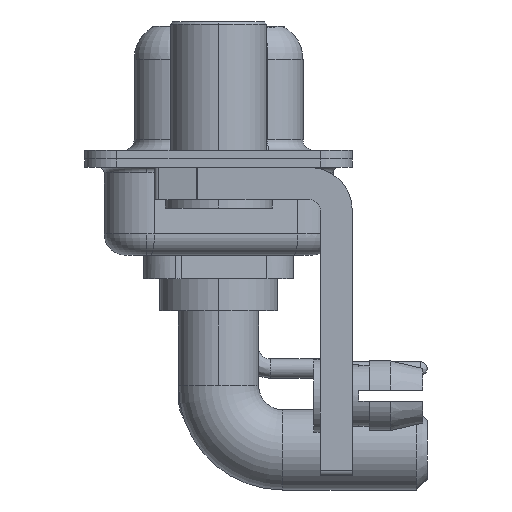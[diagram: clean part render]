
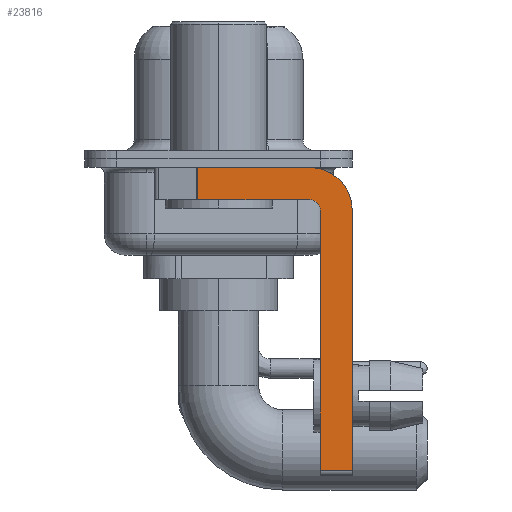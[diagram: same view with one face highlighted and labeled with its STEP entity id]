
A CAD part, left-side view. The second image highlights one B-rep face of the part: STEP entity #23816.
In plain terms, the highlighted planar face has unit normal (-1, 0, 0).
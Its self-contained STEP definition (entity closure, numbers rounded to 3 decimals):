
#2 = VERTEX_POINT ( 'NONE', #15250 ) ;
#1023 = EDGE_CURVE ( 'NONE', #3840, #24456, #2556, .T. ) ;
#1087 = LINE ( 'NONE', #9688, #4411 ) ;
#1192 = VECTOR ( 'NONE', #2834, 1000. ) ;
#2256 = CARTESIAN_POINT ( 'NONE',  ( -2.9, -4.25, -1.9 ) ) ;
#2389 = VECTOR ( 'NONE', #16974, 1000. ) ;
#2413 = VERTEX_POINT ( 'NONE', #8756 ) ;
#2511 = AXIS2_PLACEMENT_3D ( 'NONE', #18713, #27082, #12351 ) ;
#2556 = CIRCLE ( 'NONE', #6671, 2. ) ;
#2834 = DIRECTION ( 'NONE',  ( 0., -1., 0. ) ) ;
#3809 = LINE ( 'NONE', #19080, #2389 ) ;
#3840 = VERTEX_POINT ( 'NONE', #4097 ) ;
#4097 = CARTESIAN_POINT ( 'NONE',  ( -2.9, -4.25, -0.4 ) ) ;
#4411 = VECTOR ( 'NONE', #7990, 1000. ) ;
#4825 = VERTEX_POINT ( 'NONE', #17703 ) ;
#6145 = EDGE_CURVE ( 'NONE', #10726, #2413, #21607, .T. ) ;
#6243 = CARTESIAN_POINT ( 'NONE',  ( -2.9, -6.25, -2.4 ) ) ;
#6388 = DIRECTION ( 'NONE',  ( 0., 0., 1. ) ) ;
#6671 = AXIS2_PLACEMENT_3D ( 'NONE', #13459, #22083, #7351 ) ;
#7351 = DIRECTION ( 'NONE',  ( 0., 0., -1. ) ) ;
#7906 = CARTESIAN_POINT ( 'NONE',  ( -2.9, -6.25, -2.4 ) ) ;
#7990 = DIRECTION ( 'NONE',  ( 0., 0., -1. ) ) ;
#8018 = VECTOR ( 'NONE', #6388, 1000. ) ;
#8374 = DIRECTION ( 'NONE',  ( 0., 0., -1. ) ) ;
#8756 = CARTESIAN_POINT ( 'NONE',  ( -2.9, 0.978, -1.9 ) ) ;
#9688 = CARTESIAN_POINT ( 'NONE',  ( -2.9, 0.978, -1.9 ) ) ;
#10726 = VERTEX_POINT ( 'NONE', #14898 ) ;
#12304 = ORIENTED_EDGE ( 'NONE', *, *, #6145, .F. ) ;
#12351 = DIRECTION ( 'NONE',  ( 0., 0., -1. ) ) ;
#12879 = EDGE_CURVE ( 'NONE', #24753, #3840, #13444, .T. ) ;
#13284 = CARTESIAN_POINT ( 'NONE',  ( -2.9, 0.978, -0.4 ) ) ;
#13444 = LINE ( 'NONE', #19812, #1192 ) ;
#13459 = CARTESIAN_POINT ( 'NONE',  ( -2.9, -4.25, -2.4 ) ) ;
#13534 = AXIS2_PLACEMENT_3D ( 'NONE', #20669, #20394, #20259 ) ;
#14200 = FACE_OUTER_BOUND ( 'NONE', #19224, .T. ) ;
#14885 = ORIENTED_EDGE ( 'NONE', *, *, #12879, .F. ) ;
#14893 = ORIENTED_EDGE ( 'NONE', *, *, #17661, .F. ) ;
#14898 = CARTESIAN_POINT ( 'NONE',  ( -2.9, -4.25, -1.9 ) ) ;
#15250 = CARTESIAN_POINT ( 'NONE',  ( -2.9, -4.75, -14.55 ) ) ;
#15395 = DIRECTION ( 'NONE',  ( 0., 1., 0. ) ) ;
#16033 = EDGE_CURVE ( 'NONE', #2, #23342, #20977, .T. ) ;
#16467 = PLANE ( 'NONE',  #2511 ) ;
#16621 = ORIENTED_EDGE ( 'NONE', *, *, #26747, .T. ) ;
#16974 = DIRECTION ( 'NONE',  ( 0., -1., 0. ) ) ;
#17661 = EDGE_CURVE ( 'NONE', #23342, #10726, #26189, .T. ) ;
#17703 = CARTESIAN_POINT ( 'NONE',  ( -2.9, -6.25, -14.55 ) ) ;
#18713 = CARTESIAN_POINT ( 'NONE',  ( -2.9, -4.25, -2.4 ) ) ;
#18818 = VECTOR ( 'NONE', #8374, 1000. ) ;
#19080 = CARTESIAN_POINT ( 'NONE',  ( -2.9, -4.25, -14.55 ) ) ;
#19220 = ORIENTED_EDGE ( 'NONE', *, *, #1023, .F. ) ;
#19224 = EDGE_LOOP ( 'NONE', ( #14885, #16621, #12304, #14893, #25361, #25201, #24457, #19220 ) ) ;
#19266 = LINE ( 'NONE', #6243, #18818 ) ;
#19812 = CARTESIAN_POINT ( 'NONE',  ( -2.9, 3., -0.4 ) ) ;
#19819 = EDGE_CURVE ( 'NONE', #2, #4825, #3809, .T. ) ;
#20244 = VECTOR ( 'NONE', #15395, 1000. ) ;
#20259 = DIRECTION ( 'NONE',  ( 0., 0., 1. ) ) ;
#20394 = DIRECTION ( 'NONE',  ( -1., 0., 0. ) ) ;
#20669 = CARTESIAN_POINT ( 'NONE',  ( -2.9, -4.25, -2.4 ) ) ;
#20977 = LINE ( 'NONE', #25796, #8018 ) ;
#21607 = LINE ( 'NONE', #2256, #20244 ) ;
#22083 = DIRECTION ( 'NONE',  ( 1., 0., 0. ) ) ;
#23342 = VERTEX_POINT ( 'NONE', #25121 ) ;
#23816 = ADVANCED_FACE ( 'NONE', ( #14200 ), #16467, .F. ) ;
#24456 = VERTEX_POINT ( 'NONE', #7906 ) ;
#24457 = ORIENTED_EDGE ( 'NONE', *, *, #25487, .F. ) ;
#24753 = VERTEX_POINT ( 'NONE', #13284 ) ;
#25121 = CARTESIAN_POINT ( 'NONE',  ( -2.9, -4.75, -2.4 ) ) ;
#25201 = ORIENTED_EDGE ( 'NONE', *, *, #19819, .T. ) ;
#25361 = ORIENTED_EDGE ( 'NONE', *, *, #16033, .F. ) ;
#25487 = EDGE_CURVE ( 'NONE', #24456, #4825, #19266, .T. ) ;
#25796 = CARTESIAN_POINT ( 'NONE',  ( -2.9, -4.75, -14.8 ) ) ;
#26189 = CIRCLE ( 'NONE', #13534, 0.5 ) ;
#26747 = EDGE_CURVE ( 'NONE', #24753, #2413, #1087, .T. ) ;
#27082 = DIRECTION ( 'NONE',  ( 1., 0., 0. ) ) ;
